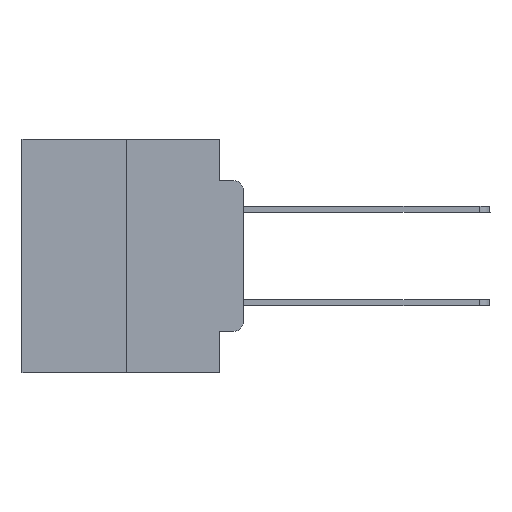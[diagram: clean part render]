
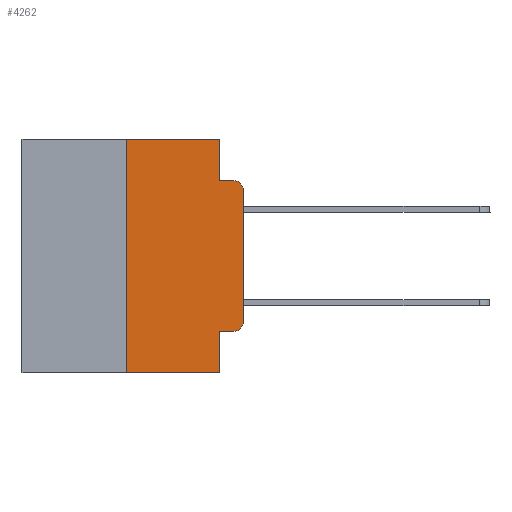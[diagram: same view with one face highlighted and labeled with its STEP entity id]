
A CAD part, left-side view. The second image highlights one B-rep face of the part: STEP entity #4262.
In plain terms, the highlighted planar face has unit normal (-1, 0, 0).
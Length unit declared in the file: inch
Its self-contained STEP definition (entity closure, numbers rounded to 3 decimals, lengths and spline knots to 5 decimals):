
#626 = CARTESIAN_POINT ( 'NONE',  ( 0., 0.02, -0.4115 ) ) ;
#756 = VERTEX_POINT ( 'NONE', #19046 ) ;
#783 = EDGE_CURVE ( 'NONE', #23058, #15265, #5636, .T. ) ;
#813 = CARTESIAN_POINT ( 'NONE',  ( 0., 0.051, -0.5 ) ) ;
#1993 = LINE ( 'NONE', #14055, #23872 ) ;
#2087 = VECTOR ( 'NONE', #14085, 39.37008 ) ;
#3397 = VECTOR ( 'NONE', #13222, 39.37008 ) ;
#3460 = LINE ( 'NONE', #8950, #8477 ) ;
#3525 = EDGE_CURVE ( 'NONE', #18215, #14081, #8183, .T. ) ;
#3842 = VERTEX_POINT ( 'NONE', #5144 ) ;
#4105 = EDGE_CURVE ( 'NONE', #15610, #14081, #9842, .T. ) ;
#4262 = ADVANCED_FACE ( 'NONE', ( #17227 ), #6436, .F. ) ;
#4772 = CARTESIAN_POINT ( 'NONE',  ( 0., 0., 0. ) ) ;
#5144 = CARTESIAN_POINT ( 'NONE',  ( 0., 0.02, -0.0885 ) ) ;
#5579 = ORIENTED_EDGE ( 'NONE', *, *, #3525, .F. ) ;
#5636 = CIRCLE ( 'NONE', #17955, 0.02 ) ;
#5962 = EDGE_CURVE ( 'NONE', #9585, #25222, #1993, .T. ) ;
#6008 = DIRECTION ( 'NONE',  ( 0., 0., -1. ) ) ;
#6094 = CARTESIAN_POINT ( 'NONE',  ( 0., 0.02, -0.1085 ) ) ;
#6168 = EDGE_CURVE ( 'NONE', #15265, #756, #19140, .T. ) ;
#6389 = EDGE_LOOP ( 'NONE', ( #7643, #11755, #12005, #9677, #25613, #27043, #13025, #5579, #21555, #26346 ) ) ;
#6436 = PLANE ( 'NONE',  #8097 ) ;
#7643 = ORIENTED_EDGE ( 'NONE', *, *, #6168, .T. ) ;
#7812 = LINE ( 'NONE', #11880, #22644 ) ;
#8097 = AXIS2_PLACEMENT_3D ( 'NONE', #8321, #15298, #15490 ) ;
#8183 = LINE ( 'NONE', #17197, #10863 ) ;
#8321 = CARTESIAN_POINT ( 'NONE',  ( 0., 0.473, 0. ) ) ;
#8477 = VECTOR ( 'NONE', #23727, 39.37008 ) ;
#8774 = VERTEX_POINT ( 'NONE', #25016 ) ;
#8950 = CARTESIAN_POINT ( 'NONE',  ( 0., 0.051, -0.4115 ) ) ;
#9519 = CARTESIAN_POINT ( 'NONE',  ( 0., 0.25, -0.5 ) ) ;
#9585 = VERTEX_POINT ( 'NONE', #11146 ) ;
#9677 = ORIENTED_EDGE ( 'NONE', *, *, #5962, .F. ) ;
#9784 = EDGE_CURVE ( 'NONE', #756, #3842, #23352, .T. ) ;
#9842 = LINE ( 'NONE', #23100, #12857 ) ;
#10863 = VECTOR ( 'NONE', #12675, 39.37008 ) ;
#11016 = CARTESIAN_POINT ( 'NONE',  ( 0., 0., -0.3915 ) ) ;
#11146 = CARTESIAN_POINT ( 'NONE',  ( 0., 0.051, 0. ) ) ;
#11476 = EDGE_CURVE ( 'NONE', #8774, #9585, #7812, .T. ) ;
#11755 = ORIENTED_EDGE ( 'NONE', *, *, #9784, .T. ) ;
#11880 = CARTESIAN_POINT ( 'NONE',  ( 0., 0.473, 0. ) ) ;
#12005 = ORIENTED_EDGE ( 'NONE', *, *, #23875, .F. ) ;
#12474 = CARTESIAN_POINT ( 'NONE',  ( 0., 0.02, -0.3915 ) ) ;
#12554 = DIRECTION ( 'NONE',  ( 0., -1., 0. ) ) ;
#12675 = DIRECTION ( 'NONE',  ( 0., 0., -1. ) ) ;
#12857 = VECTOR ( 'NONE', #12554, 39.37008 ) ;
#13025 = ORIENTED_EDGE ( 'NONE', *, *, #4105, .T. ) ;
#13222 = DIRECTION ( 'NONE',  ( 0., -1., 0. ) ) ;
#14055 = CARTESIAN_POINT ( 'NONE',  ( 0., 0.051, 0. ) ) ;
#14076 = CARTESIAN_POINT ( 'NONE',  ( 0., 0.051, -0.4115 ) ) ;
#14081 = VERTEX_POINT ( 'NONE', #813 ) ;
#14085 = DIRECTION ( 'NONE',  ( 0., 0., 1. ) ) ;
#15254 = EDGE_CURVE ( 'NONE', #18215, #23058, #3460, .T. ) ;
#15265 = VERTEX_POINT ( 'NONE', #11016 ) ;
#15298 = DIRECTION ( 'NONE',  ( 1., 0., 0. ) ) ;
#15490 = DIRECTION ( 'NONE',  ( 0., 0., -1. ) ) ;
#15523 = LINE ( 'NONE', #17170, #3397 ) ;
#15610 = VERTEX_POINT ( 'NONE', #9519 ) ;
#15902 = CARTESIAN_POINT ( 'NONE',  ( 0., 0.051, -0.0885 ) ) ;
#16166 = CARTESIAN_POINT ( 'NONE',  ( 0., 0.25, 0. ) ) ;
#17135 = VECTOR ( 'NONE', #17566, 39.37008 ) ;
#17170 = CARTESIAN_POINT ( 'NONE',  ( 0., 0.051, -0.0885 ) ) ;
#17197 = CARTESIAN_POINT ( 'NONE',  ( 0., 0.051, 0. ) ) ;
#17227 = FACE_OUTER_BOUND ( 'NONE', #6389, .T. ) ;
#17566 = DIRECTION ( 'NONE',  ( 0., 0., 1. ) ) ;
#17955 = AXIS2_PLACEMENT_3D ( 'NONE', #12474, #27495, #18959 ) ;
#18215 = VERTEX_POINT ( 'NONE', #14076 ) ;
#18914 = LINE ( 'NONE', #16166, #2087 ) ;
#18959 = DIRECTION ( 'NONE',  ( 0., 0., -1. ) ) ;
#19046 = CARTESIAN_POINT ( 'NONE',  ( 0., 0., -0.1085 ) ) ;
#19140 = LINE ( 'NONE', #4772, #17135 ) ;
#20534 = DIRECTION ( 'NONE',  ( 0., 0., -1. ) ) ;
#21044 = DIRECTION ( 'NONE',  ( -1., 0., 0. ) ) ;
#21555 = ORIENTED_EDGE ( 'NONE', *, *, #15254, .T. ) ;
#22427 = DIRECTION ( 'NONE',  ( 0., -1., 0. ) ) ;
#22644 = VECTOR ( 'NONE', #22427, 39.37008 ) ;
#22741 = EDGE_CURVE ( 'NONE', #15610, #8774, #18914, .T. ) ;
#23058 = VERTEX_POINT ( 'NONE', #626 ) ;
#23100 = CARTESIAN_POINT ( 'NONE',  ( 0., 0.473, -0.5 ) ) ;
#23352 = CIRCLE ( 'NONE', #26917, 0.02 ) ;
#23727 = DIRECTION ( 'NONE',  ( 0., -1., 0. ) ) ;
#23872 = VECTOR ( 'NONE', #20534, 39.37008 ) ;
#23875 = EDGE_CURVE ( 'NONE', #25222, #3842, #15523, .T. ) ;
#25016 = CARTESIAN_POINT ( 'NONE',  ( 0., 0.25, 0. ) ) ;
#25222 = VERTEX_POINT ( 'NONE', #15902 ) ;
#25613 = ORIENTED_EDGE ( 'NONE', *, *, #11476, .F. ) ;
#26346 = ORIENTED_EDGE ( 'NONE', *, *, #783, .T. ) ;
#26917 = AXIS2_PLACEMENT_3D ( 'NONE', #6094, #21044, #6008 ) ;
#27043 = ORIENTED_EDGE ( 'NONE', *, *, #22741, .F. ) ;
#27495 = DIRECTION ( 'NONE',  ( -1., 0., 0. ) ) ;
